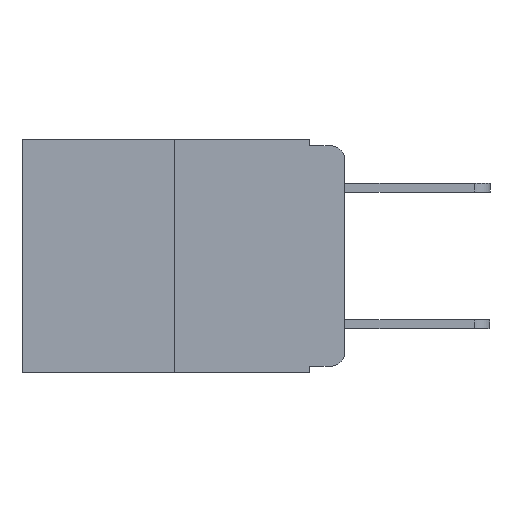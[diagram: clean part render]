
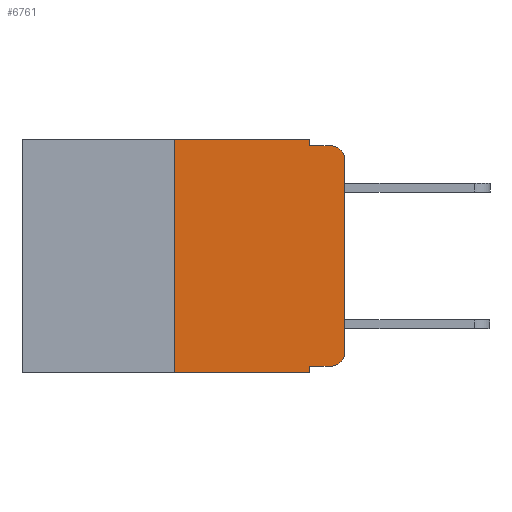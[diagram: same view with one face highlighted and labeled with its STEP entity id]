
A CAD part, left-side view. The second image highlights one B-rep face of the part: STEP entity #6761.
In plain terms, the highlighted planar face has unit normal (-1, 0, 0).
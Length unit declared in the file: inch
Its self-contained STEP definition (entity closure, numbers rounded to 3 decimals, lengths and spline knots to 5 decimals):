
#101 = ORIENTED_EDGE ( 'NONE', *, *, #17126, .T. ) ;
#150 = ORIENTED_EDGE ( 'NONE', *, *, #16075, .F. ) ;
#354 = LINE ( 'NONE', #13737, #14208 ) ;
#434 = ORIENTED_EDGE ( 'NONE', *, *, #15007, .F. ) ;
#694 = DIRECTION ( 'NONE',  ( 1., 0., 0. ) ) ;
#696 = VERTEX_POINT ( 'NONE', #18862 ) ;
#895 = ORIENTED_EDGE ( 'NONE', *, *, #9992, .F. ) ;
#1035 = ORIENTED_EDGE ( 'NONE', *, *, #13905, .F. ) ;
#1198 = VERTEX_POINT ( 'NONE', #16872 ) ;
#1270 = ORIENTED_EDGE ( 'NONE', *, *, #9675, .T. ) ;
#1721 = CARTESIAN_POINT ( 'NONE',  ( 0., 0., 0. ) ) ;
#1741 = ORIENTED_EDGE ( 'NONE', *, *, #11734, .F. ) ;
#2092 = AXIS2_PLACEMENT_3D ( 'NONE', #2470, #14896, #4405 ) ;
#2470 = CARTESIAN_POINT ( 'NONE',  ( 0., 0.02, -0.03 ) ) ;
#2756 = CARTESIAN_POINT ( 'NONE',  ( 0., 0.051, -0.333 ) ) ;
#3175 = ORIENTED_EDGE ( 'NONE', *, *, #18170, .T. ) ;
#3309 = ORIENTED_EDGE ( 'NONE', *, *, #10568, .T. ) ;
#3320 = CARTESIAN_POINT ( 'NONE',  ( 0., 0.473, -0.343 ) ) ;
#3330 = EDGE_LOOP ( 'NONE', ( #3175, #101, #150, #434, #895, #1035, #1270, #1741, #3309, #3522 ) ) ;
#3522 = ORIENTED_EDGE ( 'NONE', *, *, #9361, .T. ) ;
#3657 = DIRECTION ( 'NONE',  ( 0., 0., 1. ) ) ;
#4405 = DIRECTION ( 'NONE',  ( 0., 0., -1. ) ) ;
#4617 = CARTESIAN_POINT ( 'NONE',  ( 0., 0., -0.313 ) ) ;
#4956 = DIRECTION ( 'NONE',  ( 0., -1., 0. ) ) ;
#5196 = CARTESIAN_POINT ( 'NONE',  ( 0., 0.25, 0. ) ) ;
#5209 = VECTOR ( 'NONE', #6080, 39.37008 ) ;
#5867 = VECTOR ( 'NONE', #15542, 39.37008 ) ;
#6080 = DIRECTION ( 'NONE',  ( 0., -1., 0. ) ) ;
#6489 = LINE ( 'NONE', #20147, #5867 ) ;
#6529 = DIRECTION ( 'NONE',  ( -1., 0., 0. ) ) ;
#6761 = ADVANCED_FACE ( 'NONE', ( #21130 ), #11781, .F. ) ;
#7050 = CIRCLE ( 'NONE', #20535, 0.02 ) ;
#7146 = VERTEX_POINT ( 'NONE', #11321 ) ;
#7428 = CARTESIAN_POINT ( 'NONE',  ( 0., 0.051, -0.343 ) ) ;
#8801 = VERTEX_POINT ( 'NONE', #5196 ) ;
#9361 = EDGE_CURVE ( 'NONE', #7146, #15987, #7050, .T. ) ;
#9405 = VERTEX_POINT ( 'NONE', #2756 ) ;
#9523 = VECTOR ( 'NONE', #12675, 39.37008 ) ;
#9675 = EDGE_CURVE ( 'NONE', #696, #16941, #15761, .T. ) ;
#9709 = VECTOR ( 'NONE', #19401, 39.37008 ) ;
#9992 = EDGE_CURVE ( 'NONE', #8801, #10862, #10603, .T. ) ;
#10094 = LINE ( 'NONE', #15893, #9523 ) ;
#10216 = VECTOR ( 'NONE', #10649, 39.37008 ) ;
#10568 = EDGE_CURVE ( 'NONE', #9405, #7146, #18406, .T. ) ;
#10603 = LINE ( 'NONE', #19419, #5209 ) ;
#10649 = DIRECTION ( 'NONE',  ( 0., 0., -1. ) ) ;
#10862 = VERTEX_POINT ( 'NONE', #12458 ) ;
#11321 = CARTESIAN_POINT ( 'NONE',  ( 0., 0.02, -0.333 ) ) ;
#11438 = VECTOR ( 'NONE', #12420, 39.37008 ) ;
#11440 = LINE ( 'NONE', #1721, #19428 ) ;
#11453 = CARTESIAN_POINT ( 'NONE',  ( 0., 0.051, -0.333 ) ) ;
#11734 = EDGE_CURVE ( 'NONE', #9405, #16941, #14651, .T. ) ;
#11781 = PLANE ( 'NONE',  #13211 ) ;
#12420 = DIRECTION ( 'NONE',  ( 0., -1., 0. ) ) ;
#12458 = CARTESIAN_POINT ( 'NONE',  ( 0., 0.051, 0. ) ) ;
#12675 = DIRECTION ( 'NONE',  ( 0., 0., -1. ) ) ;
#13211 = AXIS2_PLACEMENT_3D ( 'NONE', #21160, #694, #13443 ) ;
#13443 = DIRECTION ( 'NONE',  ( 0., 0., -1. ) ) ;
#13737 = CARTESIAN_POINT ( 'NONE',  ( 0., 0.051, -0.01 ) ) ;
#13905 = EDGE_CURVE ( 'NONE', #696, #8801, #6489, .T. ) ;
#14169 = VERTEX_POINT ( 'NONE', #15950 ) ;
#14208 = VECTOR ( 'NONE', #4956, 39.37008 ) ;
#14299 = CARTESIAN_POINT ( 'NONE',  ( 0., 0., -0.03 ) ) ;
#14651 = LINE ( 'NONE', #18703, #10216 ) ;
#14896 = DIRECTION ( 'NONE',  ( -1., 0., 0. ) ) ;
#15007 = EDGE_CURVE ( 'NONE', #10862, #14169, #10094, .T. ) ;
#15542 = DIRECTION ( 'NONE',  ( 0., 0., 1. ) ) ;
#15761 = LINE ( 'NONE', #3320, #11438 ) ;
#15800 = CIRCLE ( 'NONE', #2092, 0.02 ) ;
#15893 = CARTESIAN_POINT ( 'NONE',  ( 0., 0.051, 0. ) ) ;
#15950 = CARTESIAN_POINT ( 'NONE',  ( 0., 0.051, -0.01 ) ) ;
#15987 = VERTEX_POINT ( 'NONE', #4617 ) ;
#16075 = EDGE_CURVE ( 'NONE', #14169, #1198, #354, .T. ) ;
#16640 = CARTESIAN_POINT ( 'NONE',  ( 0., 0.02, -0.313 ) ) ;
#16872 = CARTESIAN_POINT ( 'NONE',  ( 0., 0.02, -0.01 ) ) ;
#16941 = VERTEX_POINT ( 'NONE', #7428 ) ;
#17126 = EDGE_CURVE ( 'NONE', #17502, #1198, #15800, .T. ) ;
#17502 = VERTEX_POINT ( 'NONE', #14299 ) ;
#18170 = EDGE_CURVE ( 'NONE', #15987, #17502, #11440, .T. ) ;
#18227 = DIRECTION ( 'NONE',  ( 0., 0., -1. ) ) ;
#18406 = LINE ( 'NONE', #11453, #9709 ) ;
#18703 = CARTESIAN_POINT ( 'NONE',  ( 0., 0.051, 0. ) ) ;
#18862 = CARTESIAN_POINT ( 'NONE',  ( 0., 0.25, -0.343 ) ) ;
#19401 = DIRECTION ( 'NONE',  ( 0., -1., 0. ) ) ;
#19419 = CARTESIAN_POINT ( 'NONE',  ( 0., 0.473, 0. ) ) ;
#19428 = VECTOR ( 'NONE', #3657, 39.37008 ) ;
#20147 = CARTESIAN_POINT ( 'NONE',  ( 0., 0.25, 0. ) ) ;
#20535 = AXIS2_PLACEMENT_3D ( 'NONE', #16640, #6529, #18227 ) ;
#21130 = FACE_OUTER_BOUND ( 'NONE', #3330, .T. ) ;
#21160 = CARTESIAN_POINT ( 'NONE',  ( 0., 0.473, 0. ) ) ;
